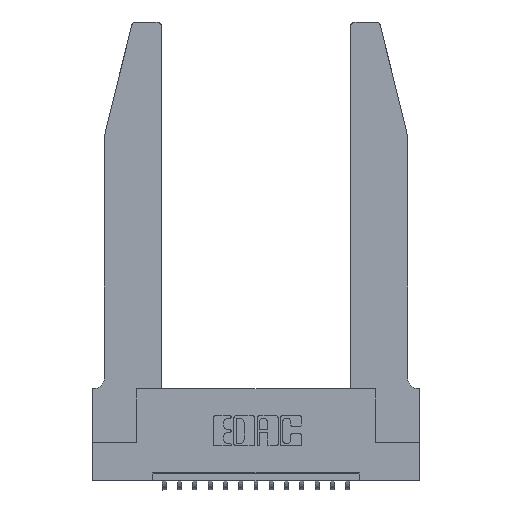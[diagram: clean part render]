
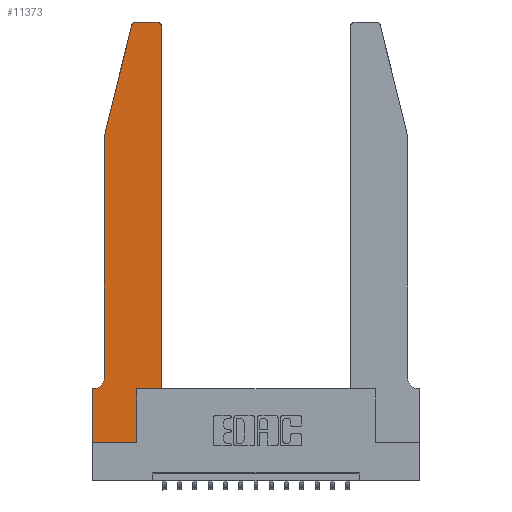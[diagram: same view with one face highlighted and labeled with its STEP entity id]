
A CAD part, top view. The second image highlights one B-rep face of the part: STEP entity #11373.
In plain terms, the highlighted planar face has unit normal (0, 0, 1).
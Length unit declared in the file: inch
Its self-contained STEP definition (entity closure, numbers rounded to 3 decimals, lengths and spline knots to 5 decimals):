
#110 = DIRECTION ( 'NONE',  ( 1., 0., 0. ) ) ;
#147 = ORIENTED_EDGE ( 'NONE', *, *, #12955, .T. ) ;
#200 = CARTESIAN_POINT ( 'NONE',  ( 0.0755, 0.35, 0.37 ) ) ;
#241 = DIRECTION ( 'NONE',  ( 0., 0., -1. ) ) ;
#431 = DIRECTION ( 'NONE',  ( 1., 0., 0. ) ) ;
#629 = VERTEX_POINT ( 'NONE', #18497 ) ;
#758 = VERTEX_POINT ( 'NONE', #15955 ) ;
#1001 = LINE ( 'NONE', #200, #2353 ) ;
#1024 = CARTESIAN_POINT ( 'NONE',  ( 0.0755, 2., 0.37 ) ) ;
#1184 = ORIENTED_EDGE ( 'NONE', *, *, #5244, .T. ) ;
#1302 = EDGE_CURVE ( 'NONE', #7906, #7697, #3403, .T. ) ;
#1306 = LINE ( 'NONE', #3395, #2895 ) ;
#1745 = VERTEX_POINT ( 'NONE', #3085 ) ;
#1808 = EDGE_CURVE ( 'NONE', #15917, #7906, #14747, .T. ) ;
#1810 = VECTOR ( 'NONE', #2455, 39.37008 ) ;
#2265 = EDGE_CURVE ( 'NONE', #9743, #3218, #12761, .T. ) ;
#2353 = VECTOR ( 'NONE', #18520, 39.37008 ) ;
#2375 = CARTESIAN_POINT ( 'NONE',  ( 0.0755, 2., 0.37 ) ) ;
#2455 = DIRECTION ( 'NONE',  ( -0.239, -0.971, 0. ) ) ;
#2542 = DIRECTION ( 'NONE',  ( 1., 0., 0. ) ) ;
#2895 = VECTOR ( 'NONE', #16323, 39.37008 ) ;
#3085 = CARTESIAN_POINT ( 'NONE',  ( 0., 0.35, 0.37 ) ) ;
#3174 = VECTOR ( 'NONE', #431, 39.37008 ) ;
#3199 = CARTESIAN_POINT ( 'NONE',  ( 0., 0., 0.37 ) ) ;
#3218 = VERTEX_POINT ( 'NONE', #17611 ) ;
#3395 = CARTESIAN_POINT ( 'NONE',  ( 0.4505, 0.35, 0.37 ) ) ;
#3403 = LINE ( 'NONE', #1024, #1810 ) ;
#3666 = CARTESIAN_POINT ( 'NONE',  ( 0.4205, 2.75, 0.37 ) ) ;
#3898 = LINE ( 'NONE', #3199, #12630 ) ;
#4074 = LINE ( 'NONE', #14017, #6814 ) ;
#4427 = EDGE_CURVE ( 'NONE', #6173, #15917, #7612, .T. ) ;
#4529 = DIRECTION ( 'NONE',  ( 0., 0., 1. ) ) ;
#4590 = DIRECTION ( 'NONE',  ( 0., 1., 0. ) ) ;
#4792 = DIRECTION ( 'NONE',  ( 0., -1., 0. ) ) ;
#5054 = CARTESIAN_POINT ( 'NONE',  ( 0.2865, 0., 0.37 ) ) ;
#5141 = ORIENTED_EDGE ( 'NONE', *, *, #14585, .T. ) ;
#5244 = EDGE_CURVE ( 'NONE', #7549, #9743, #6895, .T. ) ;
#5500 = DIRECTION ( 'NONE',  ( 0., 0., 1. ) ) ;
#5752 = CARTESIAN_POINT ( 'NONE',  ( 0., 0., 0.37 ) ) ;
#5778 = DIRECTION ( 'NONE',  ( -1., 0., 0. ) ) ;
#6173 = VERTEX_POINT ( 'NONE', #3666 ) ;
#6237 = EDGE_CURVE ( 'NONE', #7697, #758, #4074, .T. ) ;
#6369 = ORIENTED_EDGE ( 'NONE', *, *, #16178, .T. ) ;
#6480 = CARTESIAN_POINT ( 'NONE',  ( 0.0055, 0.35, 0.37 ) ) ;
#6527 = DIRECTION ( 'NONE',  ( 1., 0., 0. ) ) ;
#6814 = VECTOR ( 'NONE', #18469, 39.37008 ) ;
#6895 = LINE ( 'NONE', #15394, #17098 ) ;
#7509 = AXIS2_PLACEMENT_3D ( 'NONE', #14866, #9399, #6527 ) ;
#7549 = VERTEX_POINT ( 'NONE', #5752 ) ;
#7612 = LINE ( 'NONE', #8176, #15331 ) ;
#7697 = VERTEX_POINT ( 'NONE', #2375 ) ;
#7739 = EDGE_CURVE ( 'NONE', #8550, #6173, #8476, .T. ) ;
#7807 = CIRCLE ( 'NONE', #11312, 0.07 ) ;
#7906 = VERTEX_POINT ( 'NONE', #14310 ) ;
#7924 = EDGE_CURVE ( 'NONE', #629, #8550, #1306, .T. ) ;
#7992 = CARTESIAN_POINT ( 'NONE',  ( 0.284, 2.75, 0.37 ) ) ;
#8158 = CARTESIAN_POINT ( 'NONE',  ( 0.0055, 0.42, 0.37 ) ) ;
#8176 = CARTESIAN_POINT ( 'NONE',  ( 0.2605, 2.75, 0.37 ) ) ;
#8413 = VERTEX_POINT ( 'NONE', #6480 ) ;
#8427 = ORIENTED_EDGE ( 'NONE', *, *, #4427, .T. ) ;
#8476 = CIRCLE ( 'NONE', #12348, 0.03 ) ;
#8550 = VERTEX_POINT ( 'NONE', #17372 ) ;
#9052 = AXIS2_PLACEMENT_3D ( 'NONE', #10767, #4529, #110 ) ;
#9399 = DIRECTION ( 'NONE',  ( 0., 0., 1. ) ) ;
#9743 = VERTEX_POINT ( 'NONE', #5054 ) ;
#9822 = DIRECTION ( 'NONE',  ( -1., 0., 0. ) ) ;
#10734 = PLANE ( 'NONE',  #7509 ) ;
#10746 = EDGE_CURVE ( 'NONE', #758, #8413, #7807, .T. ) ;
#10767 = CARTESIAN_POINT ( 'NONE',  ( 0.284, 2.72, 0.37 ) ) ;
#11312 = AXIS2_PLACEMENT_3D ( 'NONE', #8158, #241, #9822 ) ;
#11373 = ADVANCED_FACE ( 'NONE', ( #13083 ), #10734, .T. ) ;
#11909 = ORIENTED_EDGE ( 'NONE', *, *, #1302, .T. ) ;
#12348 = AXIS2_PLACEMENT_3D ( 'NONE', #12611, #5500, #13928 ) ;
#12611 = CARTESIAN_POINT ( 'NONE',  ( 0.4205, 2.72, 0.37 ) ) ;
#12630 = VECTOR ( 'NONE', #4792, 39.37008 ) ;
#12761 = LINE ( 'NONE', #15743, #13218 ) ;
#12955 = EDGE_CURVE ( 'NONE', #8413, #1745, #1001, .T. ) ;
#13083 = FACE_OUTER_BOUND ( 'NONE', #13482, .T. ) ;
#13172 = ORIENTED_EDGE ( 'NONE', *, *, #10746, .T. ) ;
#13218 = VECTOR ( 'NONE', #4590, 39.37008 ) ;
#13482 = EDGE_LOOP ( 'NONE', ( #8427, #14450, #11909, #15573, #13172, #147, #5141, #1184, #17177, #6369, #14168, #14554 ) ) ;
#13928 = DIRECTION ( 'NONE',  ( 1., 0., 0. ) ) ;
#14017 = CARTESIAN_POINT ( 'NONE',  ( 0.0755, 2., 0.37 ) ) ;
#14168 = ORIENTED_EDGE ( 'NONE', *, *, #7924, .T. ) ;
#14310 = CARTESIAN_POINT ( 'NONE',  ( 0.25487, 2.72718, 0.37 ) ) ;
#14450 = ORIENTED_EDGE ( 'NONE', *, *, #1808, .T. ) ;
#14545 = LINE ( 'NONE', #16319, #3174 ) ;
#14554 = ORIENTED_EDGE ( 'NONE', *, *, #7739, .T. ) ;
#14585 = EDGE_CURVE ( 'NONE', #1745, #7549, #3898, .T. ) ;
#14747 = CIRCLE ( 'NONE', #9052, 0.03 ) ;
#14866 = CARTESIAN_POINT ( 'NONE',  ( 0., 0.35, 0.37 ) ) ;
#15331 = VECTOR ( 'NONE', #5778, 39.37008 ) ;
#15394 = CARTESIAN_POINT ( 'NONE',  ( 0., 0., 0.37 ) ) ;
#15573 = ORIENTED_EDGE ( 'NONE', *, *, #6237, .T. ) ;
#15743 = CARTESIAN_POINT ( 'NONE',  ( 0.2865, 0.35, 0.37 ) ) ;
#15917 = VERTEX_POINT ( 'NONE', #7992 ) ;
#15955 = CARTESIAN_POINT ( 'NONE',  ( 0.0755, 0.42, 0.37 ) ) ;
#16178 = EDGE_CURVE ( 'NONE', #3218, #629, #14545, .T. ) ;
#16319 = CARTESIAN_POINT ( 'NONE',  ( 0.4505, 0.35, 0.37 ) ) ;
#16323 = DIRECTION ( 'NONE',  ( 0., 1., 0. ) ) ;
#17098 = VECTOR ( 'NONE', #2542, 39.37008 ) ;
#17177 = ORIENTED_EDGE ( 'NONE', *, *, #2265, .T. ) ;
#17372 = CARTESIAN_POINT ( 'NONE',  ( 0.4505, 2.72, 0.37 ) ) ;
#17611 = CARTESIAN_POINT ( 'NONE',  ( 0.2865, 0.35, 0.37 ) ) ;
#18469 = DIRECTION ( 'NONE',  ( 0., -1., 0. ) ) ;
#18497 = CARTESIAN_POINT ( 'NONE',  ( 0.4505, 0.35, 0.37 ) ) ;
#18520 = DIRECTION ( 'NONE',  ( -1., 0., 0. ) ) ;
